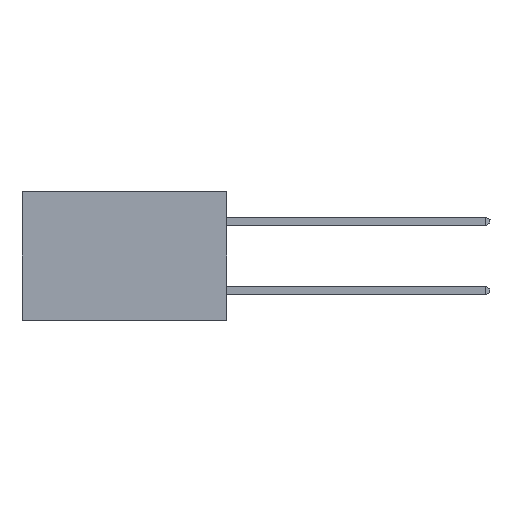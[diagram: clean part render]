
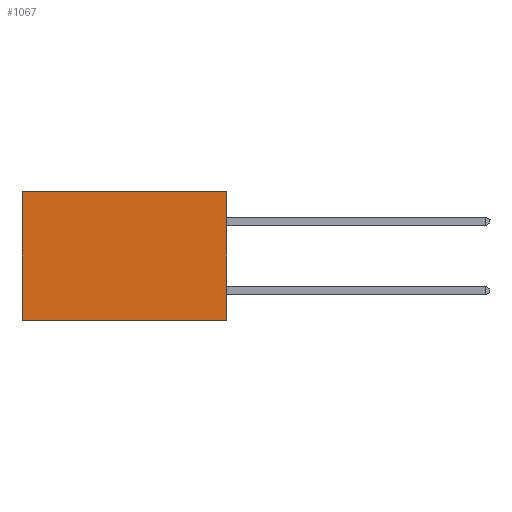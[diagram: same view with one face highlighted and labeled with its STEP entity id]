
A CAD part, left-side view. The second image highlights one B-rep face of the part: STEP entity #1067.
In plain terms, the highlighted planar face has unit normal (-1, 0, 0).
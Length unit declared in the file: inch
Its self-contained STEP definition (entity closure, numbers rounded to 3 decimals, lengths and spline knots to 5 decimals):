
#388 = LINE ( 'NONE', #2931, #3459 ) ;
#1067 = ADVANCED_FACE ( 'NONE', ( #6876 ), #17773, .F. ) ;
#1198 = VERTEX_POINT ( 'NONE', #15513 ) ;
#1721 = LINE ( 'NONE', #2865, #6270 ) ;
#2865 = CARTESIAN_POINT ( 'NONE',  ( 0.277, 0., -0.37 ) ) ;
#2931 = CARTESIAN_POINT ( 'NONE',  ( 0.277, 0.59, -0.37 ) ) ;
#2989 = ORIENTED_EDGE ( 'NONE', *, *, #11218, .T. ) ;
#3148 = ORIENTED_EDGE ( 'NONE', *, *, #18950, .F. ) ;
#3309 = EDGE_CURVE ( 'NONE', #15540, #5901, #3887, .T. ) ;
#3459 = VECTOR ( 'NONE', #4504, 39.37008 ) ;
#3761 = ORIENTED_EDGE ( 'NONE', *, *, #13324, .F. ) ;
#3772 = CARTESIAN_POINT ( 'NONE',  ( 0.277, 0., -0.37 ) ) ;
#3887 = LINE ( 'NONE', #18030, #16347 ) ;
#4031 = ORIENTED_EDGE ( 'NONE', *, *, #3309, .T. ) ;
#4504 = DIRECTION ( 'NONE',  ( 0., 0., -1. ) ) ;
#4732 = AXIS2_PLACEMENT_3D ( 'NONE', #16892, #15773, #15406 ) ;
#5901 = VERTEX_POINT ( 'NONE', #18802 ) ;
#6065 = CARTESIAN_POINT ( 'NONE',  ( 0.277, 0., -0.37 ) ) ;
#6270 = VECTOR ( 'NONE', #13438, 39.37008 ) ;
#6876 = FACE_OUTER_BOUND ( 'NONE', #15362, .T. ) ;
#7042 = VECTOR ( 'NONE', #10640, 39.37008 ) ;
#8734 = VERTEX_POINT ( 'NONE', #3772 ) ;
#10082 = CARTESIAN_POINT ( 'NONE',  ( 0.277, 0., 0. ) ) ;
#10640 = DIRECTION ( 'NONE',  ( 0., 1., 0. ) ) ;
#11069 = LINE ( 'NONE', #6065, #7042 ) ;
#11218 = EDGE_CURVE ( 'NONE', #5901, #1198, #388, .T. ) ;
#13324 = EDGE_CURVE ( 'NONE', #15540, #8734, #1721, .T. ) ;
#13438 = DIRECTION ( 'NONE',  ( 0., 0., -1. ) ) ;
#15362 = EDGE_LOOP ( 'NONE', ( #2989, #3148, #3761, #4031 ) ) ;
#15406 = DIRECTION ( 'NONE',  ( 0., 0., -1. ) ) ;
#15513 = CARTESIAN_POINT ( 'NONE',  ( 0.277, 0.59, -0.37 ) ) ;
#15540 = VERTEX_POINT ( 'NONE', #10082 ) ;
#15773 = DIRECTION ( 'NONE',  ( 1., 0., 0. ) ) ;
#16347 = VECTOR ( 'NONE', #18023, 39.37008 ) ;
#16892 = CARTESIAN_POINT ( 'NONE',  ( 0.277, 0., -0.37 ) ) ;
#17773 = PLANE ( 'NONE',  #4732 ) ;
#18023 = DIRECTION ( 'NONE',  ( 0., 1., 0. ) ) ;
#18030 = CARTESIAN_POINT ( 'NONE',  ( 0.277, 0., 0. ) ) ;
#18802 = CARTESIAN_POINT ( 'NONE',  ( 0.277, 0.59, 0. ) ) ;
#18950 = EDGE_CURVE ( 'NONE', #8734, #1198, #11069, .T. ) ;
